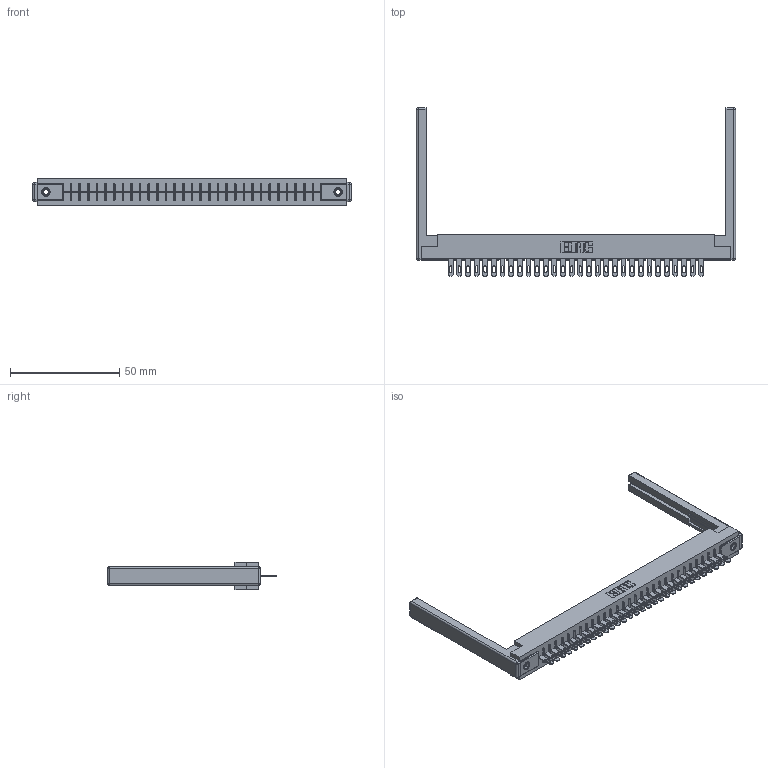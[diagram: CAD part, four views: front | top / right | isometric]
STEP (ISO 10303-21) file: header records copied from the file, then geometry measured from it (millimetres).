
FILE_DESCRIPTION (( 'STEP AP203' ), '1' );
FILE_NAME ('356-030-500-168.STEP', '2018-08-01T20:55:34', ( '' ), ( '' ), 'SwSTEP 2.0', 'SolidWorks 2016', '' );
FILE_SCHEMA (( 'CONFIG_CONTROL_DESIGN' ));
Length unit declared in the file: inch
Products named in the file (5): 306 Part_.156 Dia; 306-290-001_100; 345-250-001_345-250-001-102; 307-220-068; 356-030-500-168
Assembly tree (35 placements, depth 2):
  356-030-500-168
    306 Part_.156 Dia
    306-290-001_100  x30
    345-250-001_345-250-001-102  x2
    307-220-068  x2
Bounding box: 146.3 x 77.17 x 12.7 mm (x, y, z)
Volume: 20525.5 mm3; surface area: 21052.8 mm2
Topology: 35 solids, 35 shells, 2550 faces, 7156 edges, 4588 vertices
Faces by surface type: plane 1656, cylinder 750, sphere 128, cone 12, torus 4
Entity records: 32454 total; most frequent: CARTESIAN_POINT 5414, ORIENTED_EDGE 5358, DIRECTION 5353, EDGE_CURVE 2679, LINE 2083, VECTOR 2083, VERTEX_POINT 1696, AXIS2_PLACEMENT_3D 1635
